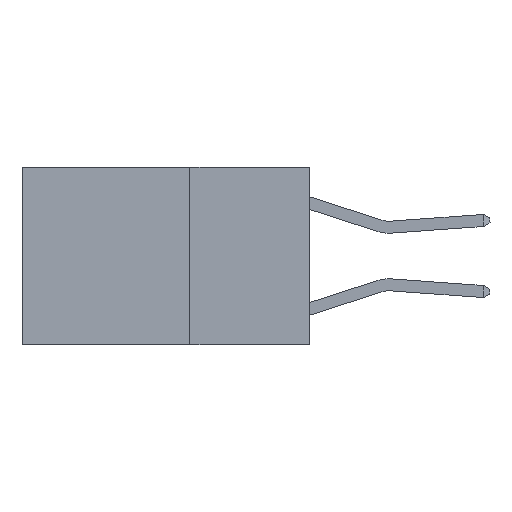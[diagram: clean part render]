
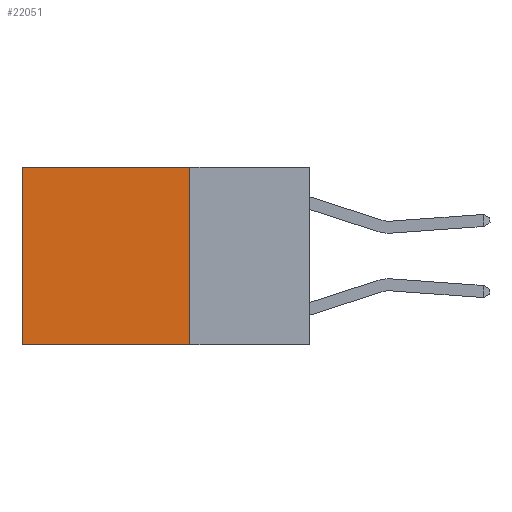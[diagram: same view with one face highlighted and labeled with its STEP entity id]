
A CAD part, left-side view. The second image highlights one B-rep face of the part: STEP entity #22051.
In plain terms, the highlighted planar face has unit normal (-1, 0, 0).
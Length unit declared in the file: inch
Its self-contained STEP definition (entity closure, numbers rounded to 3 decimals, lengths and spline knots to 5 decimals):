
#618 = CARTESIAN_POINT ( 'NONE',  ( 0.2625, 0.25, 0. ) ) ;
#2334 = EDGE_LOOP ( 'NONE', ( #19961, #7801, #8400, #11169 ) ) ;
#3286 = CARTESIAN_POINT ( 'NONE',  ( 0.2625, 0.25, 0. ) ) ;
#3818 = CARTESIAN_POINT ( 'NONE',  ( 0.2625, 0.25, 0. ) ) ;
#4714 = EDGE_CURVE ( 'NONE', #23040, #7404, #22491, .T. ) ;
#5863 = VECTOR ( 'NONE', #17018, 39.37008 ) ;
#6958 = CARTESIAN_POINT ( 'NONE',  ( 0.2625, 0.25, -0.37 ) ) ;
#7145 = CARTESIAN_POINT ( 'NONE',  ( 0.2625, 0.6, 0. ) ) ;
#7404 = VERTEX_POINT ( 'NONE', #8431 ) ;
#7801 = ORIENTED_EDGE ( 'NONE', *, *, #4714, .F. ) ;
#7803 = LINE ( 'NONE', #3286, #22531 ) ;
#8012 = FACE_OUTER_BOUND ( 'NONE', #2334, .T. ) ;
#8400 = ORIENTED_EDGE ( 'NONE', *, *, #20062, .F. ) ;
#8431 = CARTESIAN_POINT ( 'NONE',  ( 0.2625, 0.6, -0.37 ) ) ;
#8679 = AXIS2_PLACEMENT_3D ( 'NONE', #3818, #17970, #17062 ) ;
#8992 = DIRECTION ( 'NONE',  ( 0., 1., 0. ) ) ;
#9742 = EDGE_CURVE ( 'NONE', #26191, #20466, #22821, .T. ) ;
#9939 = CARTESIAN_POINT ( 'NONE',  ( 0.2625, 0.6, 0. ) ) ;
#11169 = ORIENTED_EDGE ( 'NONE', *, *, #9742, .T. ) ;
#12193 = PLANE ( 'NONE',  #8679 ) ;
#12597 = CARTESIAN_POINT ( 'NONE',  ( 0.2625, 0.25, -0.37 ) ) ;
#12602 = EDGE_CURVE ( 'NONE', #20466, #7404, #23286, .T. ) ;
#14115 = VECTOR ( 'NONE', #8992, 39.37008 ) ;
#17018 = DIRECTION ( 'NONE',  ( 0., 1., 0. ) ) ;
#17062 = DIRECTION ( 'NONE',  ( 0., 0., -1. ) ) ;
#17144 = VECTOR ( 'NONE', #22284, 39.37008 ) ;
#17970 = DIRECTION ( 'NONE',  ( 1., 0., 0. ) ) ;
#19297 = CARTESIAN_POINT ( 'NONE',  ( 0.2625, 0.25, 0. ) ) ;
#19361 = DIRECTION ( 'NONE',  ( 0., 0., -1. ) ) ;
#19961 = ORIENTED_EDGE ( 'NONE', *, *, #12602, .T. ) ;
#20062 = EDGE_CURVE ( 'NONE', #26191, #23040, #7803, .T. ) ;
#20466 = VERTEX_POINT ( 'NONE', #7145 ) ;
#22051 = ADVANCED_FACE ( 'NONE', ( #8012 ), #12193, .F. ) ;
#22284 = DIRECTION ( 'NONE',  ( 0., 0., -1. ) ) ;
#22491 = LINE ( 'NONE', #6958, #14115 ) ;
#22531 = VECTOR ( 'NONE', #19361, 39.37008 ) ;
#22821 = LINE ( 'NONE', #618, #5863 ) ;
#23040 = VERTEX_POINT ( 'NONE', #12597 ) ;
#23286 = LINE ( 'NONE', #9939, #17144 ) ;
#26191 = VERTEX_POINT ( 'NONE', #19297 ) ;
